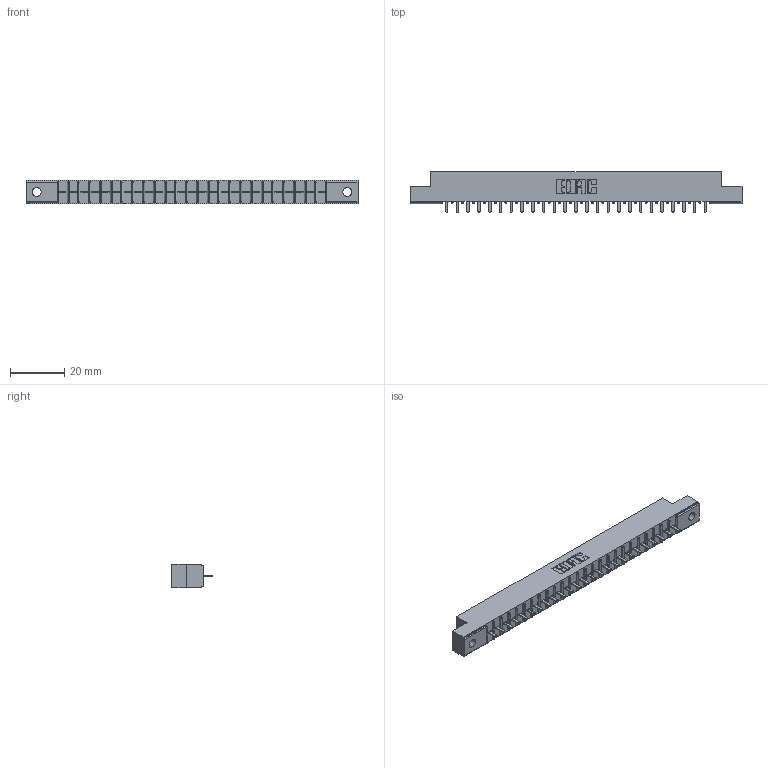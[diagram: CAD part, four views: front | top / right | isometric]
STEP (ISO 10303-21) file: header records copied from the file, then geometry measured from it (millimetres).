
FILE_DESCRIPTION (( 'STEP AP203' ), '1' );
FILE_NAME ('316-025-421-102.STEP', '2020-09-22T22:04:50', ( '' ), ( '' ), 'SwSTEP 2.0', 'SolidWorks 2020', '' );
FILE_SCHEMA (( 'CONFIG_CONTROL_DESIGN' ));
Length unit declared in the file: inch
Products named in the file (3): 306 Part_.128 Dia; 306-290-001_121; 316-025-421-102
Assembly tree (26 placements, depth 2):
  316-025-421-102
    306 Part_.128 Dia
    306-290-001_121  x25
Bounding box: 122.07 x 14.88 x 8.71 mm (x, y, z)
Volume: 8297.2 mm3; surface area: 11917.5 mm2
Topology: 26 solids, 26 shells, 1866 faces, 5241 edges, 3358 vertices
Faces by surface type: plane 1243, cylinder 523, sphere 100
Entity records: 25474 total; most frequent: CARTESIAN_POINT 4274, ORIENTED_EDGE 4234, DIRECTION 4217, EDGE_CURVE 2117, LINE 1647, VECTOR 1647, VERTEX_POINT 1342, AXIS2_PLACEMENT_3D 1285
